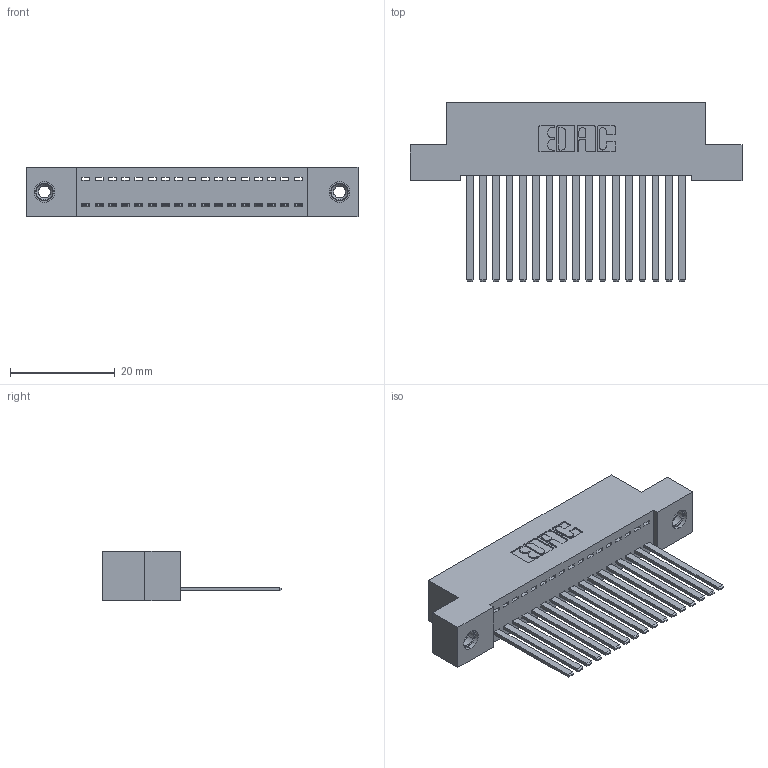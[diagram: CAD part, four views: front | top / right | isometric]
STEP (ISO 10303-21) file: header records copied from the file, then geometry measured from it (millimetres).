
FILE_DESCRIPTION (( 'STEP AP203' ), '1' );
FILE_NAME ('392-017-544-108.STEP', '2019-10-07T03:46:34', ( '' ), ( '' ), 'SwSTEP 2.0', 'SolidWorks 2016', '' );
FILE_SCHEMA (( 'CONFIG_CONTROL_DESIGN' ));
Length unit declared in the file: inch
Products named in the file (4): 392-017-544-108; 342 Part_TI; 345-292-001_345-293-144; 345-250-001_345-250-003-102
Assembly tree (20 placements, depth 2):
  392-017-544-108
    342 Part_TI
    345-292-001_345-293-144  x17
    345-250-001_345-250-003-102  x2
Bounding box: 63.5 x 34.3 x 9.4 mm (x, y, z)
Volume: 5666.8 mm3; surface area: 8432.8 mm2
Topology: 20 solids, 20 shells, 1054 faces, 3121 edges, 2050 vertices
Faces by surface type: plane 744, cylinder 294, cone 12, torus 4
Entity records: 14496 total; most frequent: CARTESIAN_POINT 2484, ORIENTED_EDGE 2430, DIRECTION 2175, EDGE_CURVE 1215, VECTOR 1071, LINE 1071, VERTEX_POINT 804, AXIS2_PLACEMENT_3D 552
